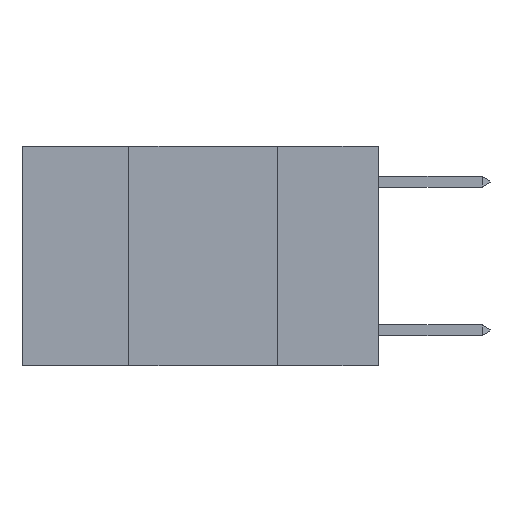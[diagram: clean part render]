
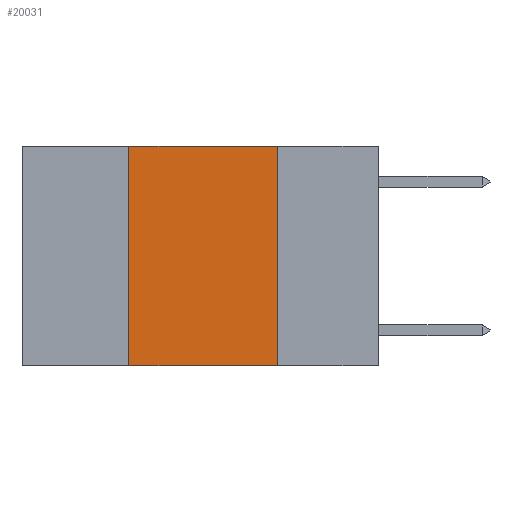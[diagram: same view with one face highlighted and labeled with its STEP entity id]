
A CAD part, left-side view. The second image highlights one B-rep face of the part: STEP entity #20031.
In plain terms, the highlighted planar face has unit normal (-1, 0, 0).
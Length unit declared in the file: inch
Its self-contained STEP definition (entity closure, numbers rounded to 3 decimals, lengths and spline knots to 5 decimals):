
#119 = VECTOR ( 'NONE', #129, 39.37008 ) ;
#129 = DIRECTION ( 'NONE',  ( 0., 0., -1. ) ) ;
#728 = VECTOR ( 'NONE', #14045, 39.37008 ) ;
#1055 = EDGE_CURVE ( 'NONE', #25642, #8159, #25193, .T. ) ;
#1142 = DIRECTION ( 'NONE',  ( 0., -1., 0. ) ) ;
#1438 = EDGE_CURVE ( 'NONE', #25642, #9622, #2395, .T. ) ;
#2395 = LINE ( 'NONE', #15379, #25228 ) ;
#4495 = LINE ( 'NONE', #19850, #119 ) ;
#4874 = VECTOR ( 'NONE', #1142, 39.37008 ) ;
#5247 = CARTESIAN_POINT ( 'NONE',  ( 0., 0.6, 0. ) ) ;
#5370 = CARTESIAN_POINT ( 'NONE',  ( 0., 0.17, 0. ) ) ;
#6416 = EDGE_CURVE ( 'NONE', #6522, #8159, #4495, .T. ) ;
#6522 = VERTEX_POINT ( 'NONE', #5370 ) ;
#7680 = CARTESIAN_POINT ( 'NONE',  ( 0., 0.6, -0.37 ) ) ;
#8159 = VERTEX_POINT ( 'NONE', #14492 ) ;
#9622 = VERTEX_POINT ( 'NONE', #27076 ) ;
#11375 = DIRECTION ( 'NONE',  ( 0., 0., 1. ) ) ;
#13024 = DIRECTION ( 'NONE',  ( 1., 0., 0. ) ) ;
#13822 = ORIENTED_EDGE ( 'NONE', *, *, #1438, .F. ) ;
#14045 = DIRECTION ( 'NONE',  ( 0., -1., 0. ) ) ;
#14492 = CARTESIAN_POINT ( 'NONE',  ( 0., 0.17, -0.37 ) ) ;
#15379 = CARTESIAN_POINT ( 'NONE',  ( 0., 0.42, 0. ) ) ;
#17513 = AXIS2_PLACEMENT_3D ( 'NONE', #19400, #13024, #28372 ) ;
#19074 = CARTESIAN_POINT ( 'NONE',  ( 0., 0.42, -0.37 ) ) ;
#19247 = PLANE ( 'NONE',  #17513 ) ;
#19400 = CARTESIAN_POINT ( 'NONE',  ( 0., 0.6, 0. ) ) ;
#19850 = CARTESIAN_POINT ( 'NONE',  ( 0., 0.17, 0. ) ) ;
#20031 = ADVANCED_FACE ( 'NONE', ( #21689 ), #19247, .F. ) ;
#20563 = LINE ( 'NONE', #5247, #728 ) ;
#21689 = FACE_OUTER_BOUND ( 'NONE', #22972, .T. ) ;
#21793 = ORIENTED_EDGE ( 'NONE', *, *, #25127, .F. ) ;
#22972 = EDGE_LOOP ( 'NONE', ( #26681, #21793, #13822, #26834 ) ) ;
#25127 = EDGE_CURVE ( 'NONE', #9622, #6522, #20563, .T. ) ;
#25193 = LINE ( 'NONE', #7680, #4874 ) ;
#25228 = VECTOR ( 'NONE', #11375, 39.37008 ) ;
#25642 = VERTEX_POINT ( 'NONE', #19074 ) ;
#26681 = ORIENTED_EDGE ( 'NONE', *, *, #6416, .F. ) ;
#26834 = ORIENTED_EDGE ( 'NONE', *, *, #1055, .T. ) ;
#27076 = CARTESIAN_POINT ( 'NONE',  ( 0., 0.42, 0. ) ) ;
#28372 = DIRECTION ( 'NONE',  ( 0., 0., -1. ) ) ;
